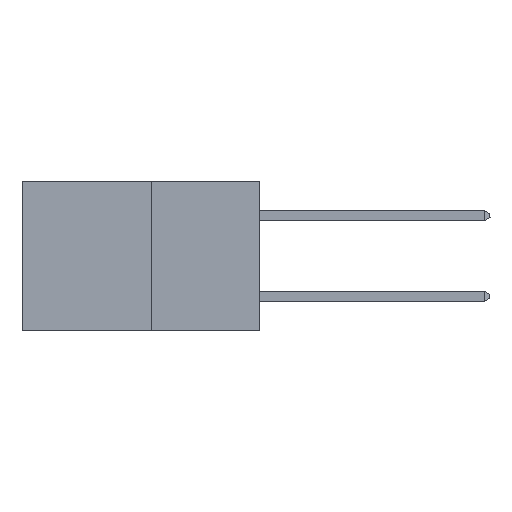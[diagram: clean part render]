
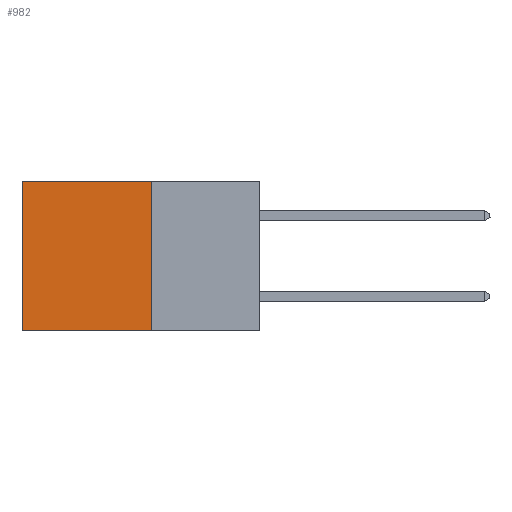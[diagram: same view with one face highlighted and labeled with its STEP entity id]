
A CAD part, left-side view. The second image highlights one B-rep face of the part: STEP entity #982.
In plain terms, the highlighted planar face has unit normal (-1, 0, 0).
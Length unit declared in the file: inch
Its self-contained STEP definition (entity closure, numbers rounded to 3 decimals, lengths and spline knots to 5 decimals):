
#817 = PLANE ( 'NONE',  #12074 ) ;
#982 = ADVANCED_FACE ( 'NONE', ( #13479 ), #817, .F. ) ;
#1088 = DIRECTION ( 'NONE',  ( 1., 0., 0. ) ) ;
#1145 = DIRECTION ( 'NONE',  ( 0., 0., -1. ) ) ;
#1254 = VECTOR ( 'NONE', #28837, 39.37008 ) ;
#1820 = CARTESIAN_POINT ( 'NONE',  ( 0.277, 0.27, -0.37 ) ) ;
#2306 = DIRECTION ( 'NONE',  ( 0., 0., -1. ) ) ;
#3307 = ORIENTED_EDGE ( 'NONE', *, *, #9843, .F. ) ;
#4563 = CARTESIAN_POINT ( 'NONE',  ( 0.277, 0.27, -0.37 ) ) ;
#5289 = DIRECTION ( 'NONE',  ( 0., 1., 0. ) ) ;
#6488 = EDGE_CURVE ( 'NONE', #13616, #8563, #19275, .T. ) ;
#8563 = VERTEX_POINT ( 'NONE', #23137 ) ;
#8672 = EDGE_CURVE ( 'NONE', #28756, #20606, #9445, .T. ) ;
#8733 = VECTOR ( 'NONE', #5289, 39.37008 ) ;
#8986 = EDGE_CURVE ( 'NONE', #8563, #20606, #13043, .T. ) ;
#9061 = CARTESIAN_POINT ( 'NONE',  ( 0.277, 0.59, -0.37 ) ) ;
#9424 = CARTESIAN_POINT ( 'NONE',  ( 0.277, 0.27, 0. ) ) ;
#9445 = LINE ( 'NONE', #16608, #8733 ) ;
#9843 = EDGE_CURVE ( 'NONE', #13616, #28756, #26325, .T. ) ;
#12074 = AXIS2_PLACEMENT_3D ( 'NONE', #1820, #1088, #1145 ) ;
#13043 = LINE ( 'NONE', #26514, #24266 ) ;
#13479 = FACE_OUTER_BOUND ( 'NONE', #25249, .T. ) ;
#13616 = VERTEX_POINT ( 'NONE', #9424 ) ;
#13703 = ORIENTED_EDGE ( 'NONE', *, *, #8986, .T. ) ;
#16608 = CARTESIAN_POINT ( 'NONE',  ( 0.277, 0.27, -0.37 ) ) ;
#17852 = ORIENTED_EDGE ( 'NONE', *, *, #6488, .T. ) ;
#18113 = CARTESIAN_POINT ( 'NONE',  ( 0.277, 0.27, -0.37 ) ) ;
#19275 = LINE ( 'NONE', #28831, #1254 ) ;
#20606 = VERTEX_POINT ( 'NONE', #9061 ) ;
#22796 = ORIENTED_EDGE ( 'NONE', *, *, #8672, .F. ) ;
#23137 = CARTESIAN_POINT ( 'NONE',  ( 0.277, 0.59, 0. ) ) ;
#24266 = VECTOR ( 'NONE', #28736, 39.37008 ) ;
#25249 = EDGE_LOOP ( 'NONE', ( #13703, #22796, #3307, #17852 ) ) ;
#25618 = VECTOR ( 'NONE', #2306, 39.37008 ) ;
#26325 = LINE ( 'NONE', #18113, #25618 ) ;
#26514 = CARTESIAN_POINT ( 'NONE',  ( 0.277, 0.59, -0.37 ) ) ;
#28736 = DIRECTION ( 'NONE',  ( 0., 0., -1. ) ) ;
#28756 = VERTEX_POINT ( 'NONE', #4563 ) ;
#28831 = CARTESIAN_POINT ( 'NONE',  ( 0.277, 0.27, 0. ) ) ;
#28837 = DIRECTION ( 'NONE',  ( 0., 1., 0. ) ) ;
